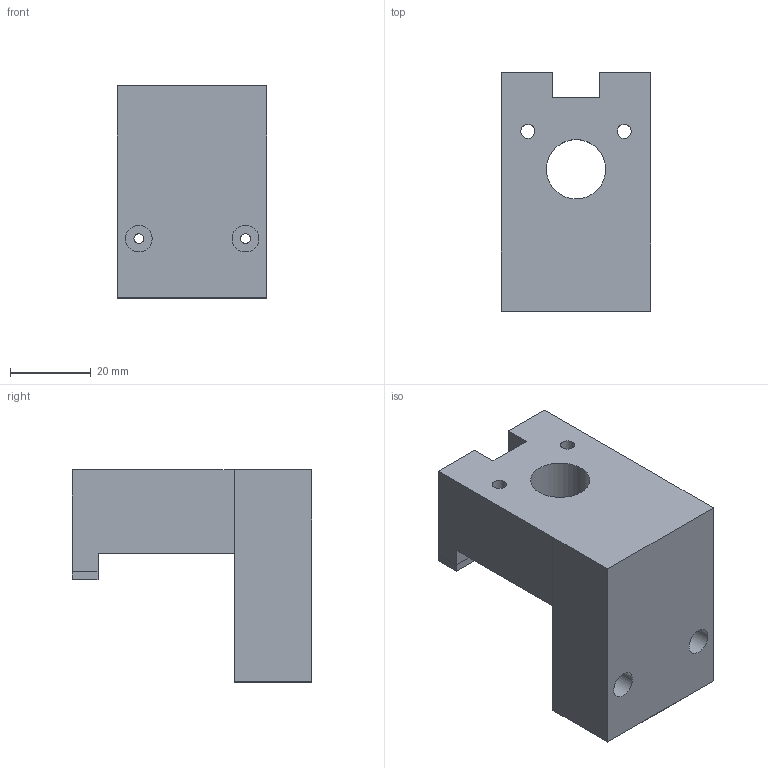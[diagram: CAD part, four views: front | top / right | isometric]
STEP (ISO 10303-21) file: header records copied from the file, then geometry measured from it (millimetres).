
FILE_DESCRIPTION(('FreeCAD Model'),'2;1');
FILE_NAME('barrel retainer.step', '2015-07-10T13:08:31',('Author'),(''), 'Open CASCADE STEP processor 6.8','FreeCAD','Unknown');
FILE_SCHEMA(('AUTOMOTIVE_DESIGN_CC2 { 1 2 10303 214 -1 1 5 4 }'));
Length unit declared in the file: millimetre
Products named in the file (1): Fusion
Bounding box: 37.11 x 59.2 x 52.56 mm (x, y, z)
Volume: 62982.3 mm3; surface area: 14231.8 mm2
Topology: 1 solids, 1 shells, 61 faces, 166 edges, 113 vertices
Faces by surface type: plane 53, cylinder 8
Full cylindrical faces by diameter (mm): 2.4 x2, 3.5 x2, 6.6 x2, 14.684 x2
Entity records: 4153 total; most frequent: CARTESIAN_POINT 794, DIRECTION 612, LINE 424, VECTOR 424, ORIENTED_EDGE 332, PCURVE 332, DEFINITIONAL_REPRESENTATION 332, EDGE_CURVE 166
